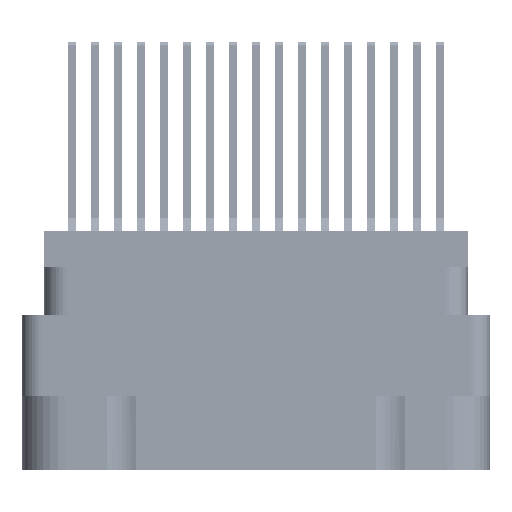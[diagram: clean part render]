
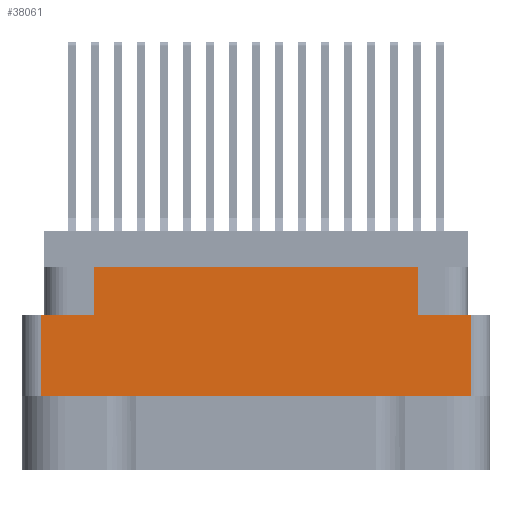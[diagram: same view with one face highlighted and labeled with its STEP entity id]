
A CAD part, left-side view. The second image highlights one B-rep face of the part: STEP entity #38061.
In plain terms, the highlighted planar face has unit normal (-1, 0, 0).
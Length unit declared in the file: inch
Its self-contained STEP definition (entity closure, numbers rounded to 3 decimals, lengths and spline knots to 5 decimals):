
#201 = DIRECTION ( 'NONE',  ( 0., 0., 1. ) ) ;
#3533 = CARTESIAN_POINT ( 'NONE',  ( -1.375, 0.5285, -0.274 ) ) ;
#4437 = ORIENTED_EDGE ( 'NONE', *, *, #82309, .T. ) ;
#7504 = ORIENTED_EDGE ( 'NONE', *, *, #68385, .T. ) ;
#8590 = CARTESIAN_POINT ( 'NONE',  ( -1.375, 0., -0.54 ) ) ;
#11367 = CARTESIAN_POINT ( 'NONE',  ( -1.375, 0.7005, -0.274 ) ) ;
#12951 = CARTESIAN_POINT ( 'NONE',  ( -1.375, -0.5285, -0.274 ) ) ;
#15921 = LINE ( 'NONE', #3533, #48638 ) ;
#19303 = DIRECTION ( 'NONE',  ( 0., -1., 0. ) ) ;
#19348 = CARTESIAN_POINT ( 'NONE',  ( -1.375, 0., -0.274 ) ) ;
#21390 = DIRECTION ( 'NONE',  ( 0., -1., 0. ) ) ;
#21858 = ORIENTED_EDGE ( 'NONE', *, *, #28196, .F. ) ;
#24031 = DIRECTION ( 'NONE',  ( -1., 0., 0. ) ) ;
#25151 = ORIENTED_EDGE ( 'NONE', *, *, #84719, .F. ) ;
#26026 = CARTESIAN_POINT ( 'NONE',  ( -1.375, 0.7625, -0.117 ) ) ;
#28196 = EDGE_CURVE ( 'NONE', #46731, #71762, #35708, .T. ) ;
#28969 = FACE_OUTER_BOUND ( 'NONE', #71741, .T. ) ;
#29736 = EDGE_CURVE ( 'NONE', #71762, #39646, #15921, .T. ) ;
#31324 = CARTESIAN_POINT ( 'NONE',  ( -1.375, -0.7625, -0.78 ) ) ;
#31638 = CARTESIAN_POINT ( 'NONE',  ( -1.375, 0.5285, -0.274 ) ) ;
#31987 = VERTEX_POINT ( 'NONE', #39620 ) ;
#32391 = ORIENTED_EDGE ( 'NONE', *, *, #62758, .F. ) ;
#33373 = DIRECTION ( 'NONE',  ( 0., -1., 0. ) ) ;
#34788 = VERTEX_POINT ( 'NONE', #43256 ) ;
#34865 = CARTESIAN_POINT ( 'NONE',  ( -1.375, -0.7005, -0.78 ) ) ;
#35708 = LINE ( 'NONE', #60005, #68681 ) ;
#36465 = ORIENTED_EDGE ( 'NONE', *, *, #55406, .T. ) ;
#38061 = ADVANCED_FACE ( 'NONE', ( #28969 ), #79349, .T. ) ;
#38697 = VECTOR ( 'NONE', #19303, 39.37008 ) ;
#38699 = VECTOR ( 'NONE', #82795, 39.37008 ) ;
#39620 = CARTESIAN_POINT ( 'NONE',  ( -1.375, 0.7005, -0.54 ) ) ;
#39646 = VERTEX_POINT ( 'NONE', #87068 ) ;
#40566 = CARTESIAN_POINT ( 'NONE',  ( -1.375, 0.7005, -0.78 ) ) ;
#40698 = VECTOR ( 'NONE', #201, 39.37008 ) ;
#43075 = LINE ( 'NONE', #40566, #38699 ) ;
#43256 = CARTESIAN_POINT ( 'NONE',  ( -1.375, -0.5285, -0.117 ) ) ;
#45113 = LINE ( 'NONE', #83252, #40698 ) ;
#46370 = ORIENTED_EDGE ( 'NONE', *, *, #29736, .F. ) ;
#46731 = VERTEX_POINT ( 'NONE', #11367 ) ;
#48638 = VECTOR ( 'NONE', #65814, 39.37008 ) ;
#49252 = VERTEX_POINT ( 'NONE', #79771 ) ;
#53102 = EDGE_CURVE ( 'NONE', #74181, #49252, #82914, .T. ) ;
#55406 = EDGE_CURVE ( 'NONE', #46731, #31987, #43075, .T. ) ;
#56720 = CARTESIAN_POINT ( 'NONE',  ( -1.375, -0.7005, -0.54 ) ) ;
#58751 = VERTEX_POINT ( 'NONE', #12951 ) ;
#59136 = DIRECTION ( 'NONE',  ( 0., 0., 1. ) ) ;
#59401 = AXIS2_PLACEMENT_3D ( 'NONE', #31324, #24031, #59136 ) ;
#60005 = CARTESIAN_POINT ( 'NONE',  ( -1.375, 0., -0.274 ) ) ;
#62758 = EDGE_CURVE ( 'NONE', #58751, #49252, #84497, .T. ) ;
#65814 = DIRECTION ( 'NONE',  ( 0., 0., 1. ) ) ;
#66115 = LINE ( 'NONE', #26026, #38697 ) ;
#68385 = EDGE_CURVE ( 'NONE', #31987, #74181, #74075, .T. ) ;
#68681 = VECTOR ( 'NONE', #73182, 39.37008 ) ;
#70322 = VECTOR ( 'NONE', #33373, 39.37008 ) ;
#71741 = EDGE_LOOP ( 'NONE', ( #21858, #36465, #7504, #90466, #32391, #4437, #25151, #46370 ) ) ;
#71762 = VERTEX_POINT ( 'NONE', #31638 ) ;
#73182 = DIRECTION ( 'NONE',  ( 0., -1., 0. ) ) ;
#74075 = LINE ( 'NONE', #8590, #88206 ) ;
#74181 = VERTEX_POINT ( 'NONE', #56720 ) ;
#79349 = PLANE ( 'NONE',  #59401 ) ;
#79771 = CARTESIAN_POINT ( 'NONE',  ( -1.375, -0.7005, -0.274 ) ) ;
#82309 = EDGE_CURVE ( 'NONE', #58751, #34788, #45113, .T. ) ;
#82795 = DIRECTION ( 'NONE',  ( 0., 0., -1. ) ) ;
#82914 = LINE ( 'NONE', #34865, #90529 ) ;
#83252 = CARTESIAN_POINT ( 'NONE',  ( -1.375, -0.5285, -0.274 ) ) ;
#83820 = DIRECTION ( 'NONE',  ( 0., 0., 1. ) ) ;
#84497 = LINE ( 'NONE', #19348, #70322 ) ;
#84719 = EDGE_CURVE ( 'NONE', #39646, #34788, #66115, .T. ) ;
#87068 = CARTESIAN_POINT ( 'NONE',  ( -1.375, 0.5285, -0.117 ) ) ;
#88206 = VECTOR ( 'NONE', #21390, 39.37008 ) ;
#90466 = ORIENTED_EDGE ( 'NONE', *, *, #53102, .T. ) ;
#90529 = VECTOR ( 'NONE', #83820, 39.37008 ) ;
